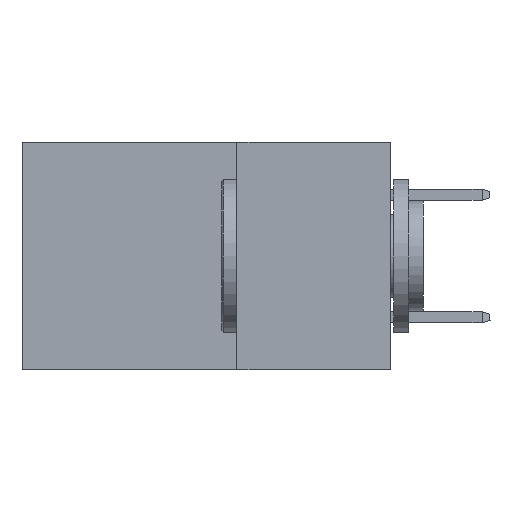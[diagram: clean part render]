
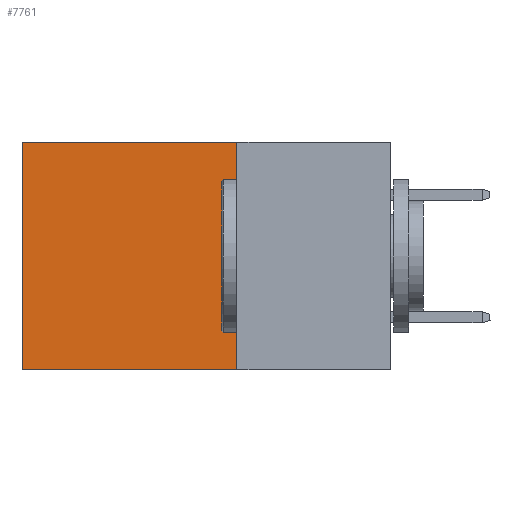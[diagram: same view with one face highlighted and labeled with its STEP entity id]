
A CAD part, left-side view. The second image highlights one B-rep face of the part: STEP entity #7761.
In plain terms, the highlighted planar face has unit normal (-1, 0, 0).
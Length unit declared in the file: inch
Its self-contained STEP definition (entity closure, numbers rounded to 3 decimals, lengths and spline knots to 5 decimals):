
#447 = VECTOR ( 'NONE', #12086, 39.37008 ) ;
#1790 = CARTESIAN_POINT ( 'NONE',  ( 0.2875, 0.25, -0.37 ) ) ;
#2634 = ORIENTED_EDGE ( 'NONE', *, *, #28618, .T. ) ;
#4268 = EDGE_CURVE ( 'NONE', #23212, #17985, #21333, .T. ) ;
#4819 = DIRECTION ( 'NONE',  ( 0., 1., 0. ) ) ;
#7021 = DIRECTION ( 'NONE',  ( 0., 0., -1. ) ) ;
#7587 = CARTESIAN_POINT ( 'NONE',  ( 0.2875, 0.6, 0. ) ) ;
#7761 = ADVANCED_FACE ( 'NONE', ( #22590 ), #11947, .F. ) ;
#8086 = CARTESIAN_POINT ( 'NONE',  ( 0.2875, 0.6, 0. ) ) ;
#8746 = ORIENTED_EDGE ( 'NONE', *, *, #17292, .F. ) ;
#8939 = ORIENTED_EDGE ( 'NONE', *, *, #9494, .F. ) ;
#9494 = EDGE_CURVE ( 'NONE', #23212, #30344, #25794, .T. ) ;
#9569 = CARTESIAN_POINT ( 'NONE',  ( 0.2875, 0.25, 0. ) ) ;
#9799 = VERTEX_POINT ( 'NONE', #12421 ) ;
#11947 = PLANE ( 'NONE',  #22030 ) ;
#12086 = DIRECTION ( 'NONE',  ( 0., 0., -1. ) ) ;
#12362 = CARTESIAN_POINT ( 'NONE',  ( 0.2875, 0.25, 0. ) ) ;
#12421 = CARTESIAN_POINT ( 'NONE',  ( 0.2875, 0.6, -0.37 ) ) ;
#12584 = EDGE_LOOP ( 'NONE', ( #2634, #8746, #8939, #15575 ) ) ;
#13262 = VECTOR ( 'NONE', #4819, 39.37008 ) ;
#14208 = CARTESIAN_POINT ( 'NONE',  ( 0.2875, 0.25, 0. ) ) ;
#15575 = ORIENTED_EDGE ( 'NONE', *, *, #4268, .T. ) ;
#17100 = DIRECTION ( 'NONE',  ( 1., 0., 0. ) ) ;
#17292 = EDGE_CURVE ( 'NONE', #30344, #9799, #28731, .T. ) ;
#17985 = VERTEX_POINT ( 'NONE', #8086 ) ;
#18827 = VECTOR ( 'NONE', #7021, 39.37008 ) ;
#20657 = LINE ( 'NONE', #7587, #447 ) ;
#21333 = LINE ( 'NONE', #14208, #13262 ) ;
#22030 = AXIS2_PLACEMENT_3D ( 'NONE', #12362, #17100, #28797 ) ;
#22590 = FACE_OUTER_BOUND ( 'NONE', #12584, .T. ) ;
#23212 = VERTEX_POINT ( 'NONE', #30418 ) ;
#24562 = DIRECTION ( 'NONE',  ( 0., 1., 0. ) ) ;
#25794 = LINE ( 'NONE', #9569, #18827 ) ;
#26824 = CARTESIAN_POINT ( 'NONE',  ( 0.2875, 0.25, -0.37 ) ) ;
#27282 = VECTOR ( 'NONE', #24562, 39.37008 ) ;
#28618 = EDGE_CURVE ( 'NONE', #17985, #9799, #20657, .T. ) ;
#28731 = LINE ( 'NONE', #26824, #27282 ) ;
#28797 = DIRECTION ( 'NONE',  ( 0., 0., -1. ) ) ;
#30344 = VERTEX_POINT ( 'NONE', #1790 ) ;
#30418 = CARTESIAN_POINT ( 'NONE',  ( 0.2875, 0.25, 0. ) ) ;
